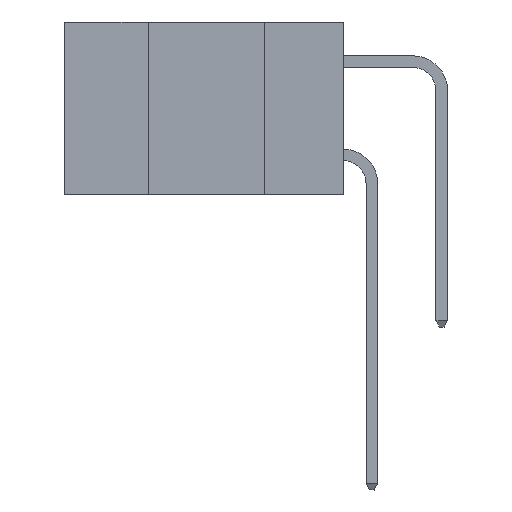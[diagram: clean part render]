
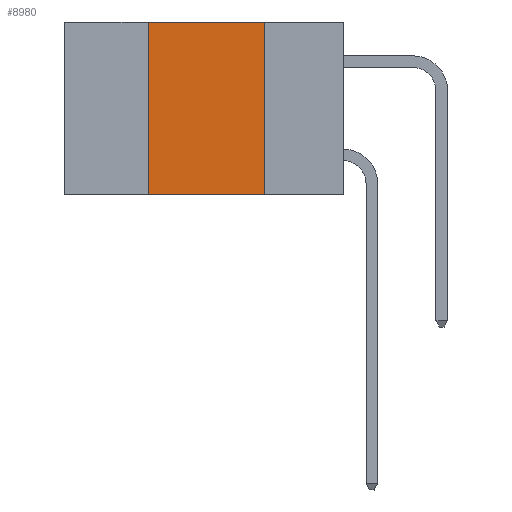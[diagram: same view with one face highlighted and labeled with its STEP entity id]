
A CAD part, left-side view. The second image highlights one B-rep face of the part: STEP entity #8980.
In plain terms, the highlighted planar face has unit normal (-1, 0, 0).
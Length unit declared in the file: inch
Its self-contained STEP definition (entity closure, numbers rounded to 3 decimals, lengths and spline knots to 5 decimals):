
#628 = AXIS2_PLACEMENT_3D ( 'NONE', #7233, #7187, #7168 ) ;
#2325 = CARTESIAN_POINT ( 'NONE',  ( 0., 0.42, -0.37 ) ) ;
#4252 = ORIENTED_EDGE ( 'NONE', *, *, #13982, .F. ) ;
#4517 = ORIENTED_EDGE ( 'NONE', *, *, #13673, .F. ) ;
#6305 = FACE_OUTER_BOUND ( 'NONE', #14995, .T. ) ;
#6418 = ORIENTED_EDGE ( 'NONE', *, *, #10854, .T. ) ;
#6735 = DIRECTION ( 'NONE',  ( 0., 0., 1. ) ) ;
#6932 = DIRECTION ( 'NONE',  ( 0., 0., -1. ) ) ;
#7091 = LINE ( 'NONE', #19500, #18670 ) ;
#7168 = DIRECTION ( 'NONE',  ( 0., 0., -1. ) ) ;
#7187 = DIRECTION ( 'NONE',  ( 1., 0., 0. ) ) ;
#7231 = VECTOR ( 'NONE', #6735, 39.37008 ) ;
#7233 = CARTESIAN_POINT ( 'NONE',  ( 0., 0.6, 0. ) ) ;
#7343 = PLANE ( 'NONE',  #628 ) ;
#7911 = CARTESIAN_POINT ( 'NONE',  ( 0., 0.17, -0.37 ) ) ;
#7960 = CARTESIAN_POINT ( 'NONE',  ( 0., 0.17, 0. ) ) ;
#8980 = ADVANCED_FACE ( 'NONE', ( #6305 ), #7343, .F. ) ;
#9321 = VECTOR ( 'NONE', #18133, 39.37008 ) ;
#10389 = VECTOR ( 'NONE', #6932, 39.37008 ) ;
#10854 = EDGE_CURVE ( 'NONE', #12759, #11823, #7091, .T. ) ;
#11809 = CARTESIAN_POINT ( 'NONE',  ( 0., 0.42, 0. ) ) ;
#11823 = VERTEX_POINT ( 'NONE', #7911 ) ;
#12034 = CARTESIAN_POINT ( 'NONE',  ( 0., 0.6, 0. ) ) ;
#12759 = VERTEX_POINT ( 'NONE', #2325 ) ;
#13550 = DIRECTION ( 'NONE',  ( 0., -1., 0. ) ) ;
#13673 = EDGE_CURVE ( 'NONE', #19406, #14542, #17458, .T. ) ;
#13982 = EDGE_CURVE ( 'NONE', #12759, #19406, #16248, .T. ) ;
#14307 = CARTESIAN_POINT ( 'NONE',  ( 0., 0.42, 0. ) ) ;
#14496 = LINE ( 'NONE', #17538, #10389 ) ;
#14542 = VERTEX_POINT ( 'NONE', #7960 ) ;
#14995 = EDGE_LOOP ( 'NONE', ( #19019, #4517, #4252, #6418 ) ) ;
#16001 = EDGE_CURVE ( 'NONE', #14542, #11823, #14496, .T. ) ;
#16248 = LINE ( 'NONE', #14307, #7231 ) ;
#17458 = LINE ( 'NONE', #12034, #9321 ) ;
#17538 = CARTESIAN_POINT ( 'NONE',  ( 0., 0.17, 0. ) ) ;
#18133 = DIRECTION ( 'NONE',  ( 0., -1., 0. ) ) ;
#18670 = VECTOR ( 'NONE', #13550, 39.37008 ) ;
#19019 = ORIENTED_EDGE ( 'NONE', *, *, #16001, .F. ) ;
#19406 = VERTEX_POINT ( 'NONE', #11809 ) ;
#19500 = CARTESIAN_POINT ( 'NONE',  ( 0., 0.6, -0.37 ) ) ;
